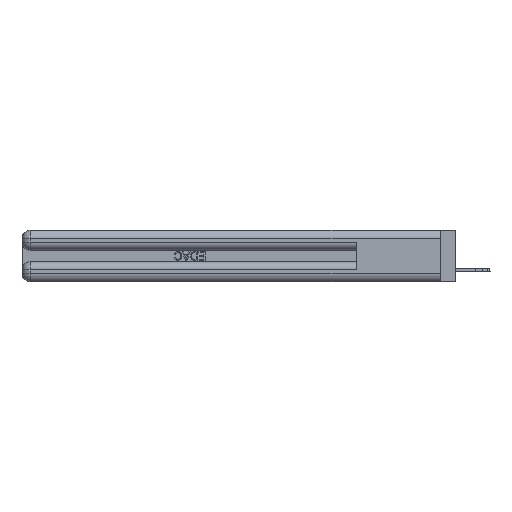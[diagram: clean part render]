
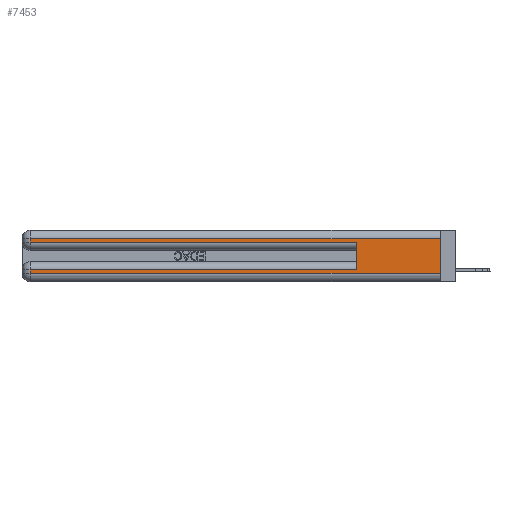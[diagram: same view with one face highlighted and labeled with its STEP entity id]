
A CAD part, left-side view. The second image highlights one B-rep face of the part: STEP entity #7453.
In plain terms, the highlighted planar face has unit normal (-1, 0, 0).
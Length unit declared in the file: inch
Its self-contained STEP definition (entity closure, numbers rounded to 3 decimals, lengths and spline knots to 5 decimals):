
#379 = CARTESIAN_POINT ( 'NONE',  ( 0., 2.94, 0.37 ) ) ;
#559 = VECTOR ( 'NONE', #15615, 39.37008 ) ;
#727 = EDGE_CURVE ( 'NONE', #10303, #22955, #10656, .T. ) ;
#872 = ORIENTED_EDGE ( 'NONE', *, *, #24029, .T. ) ;
#1413 = CARTESIAN_POINT ( 'NONE',  ( 0., 0.6, 0.285 ) ) ;
#3021 = PLANE ( 'NONE',  #16081 ) ;
#3817 = CARTESIAN_POINT ( 'NONE',  ( 0., 0., 0.085 ) ) ;
#3890 = EDGE_CURVE ( 'NONE', #19406, #32691, #26580, .T. ) ;
#3909 = DIRECTION ( 'NONE',  ( 0., 0., -1. ) ) ;
#5257 = LINE ( 'NONE', #3817, #559 ) ;
#7390 = VECTOR ( 'NONE', #3909, 39.37008 ) ;
#7453 = ADVANCED_FACE ( 'NONE', ( #27295 ), #3021, .F. ) ;
#7505 = CARTESIAN_POINT ( 'NONE',  ( 0., 0.6, 0.085 ) ) ;
#8037 = VECTOR ( 'NONE', #27867, 39.37008 ) ;
#9003 = ORIENTED_EDGE ( 'NONE', *, *, #3890, .T. ) ;
#9151 = CARTESIAN_POINT ( 'NONE',  ( 0., 0., 0.37 ) ) ;
#9726 = VECTOR ( 'NONE', #36143, 39.37008 ) ;
#10303 = VERTEX_POINT ( 'NONE', #33658 ) ;
#10656 = LINE ( 'NONE', #9151, #18634 ) ;
#11494 = EDGE_CURVE ( 'NONE', #32691, #19938, #33263, .T. ) ;
#11659 = ORIENTED_EDGE ( 'NONE', *, *, #15062, .F. ) ;
#12539 = DIRECTION ( 'NONE',  ( 0., -1., 0. ) ) ;
#13147 = VECTOR ( 'NONE', #12539, 39.37008 ) ;
#13221 = LINE ( 'NONE', #14712, #25880 ) ;
#13376 = VECTOR ( 'NONE', #16590, 39.37008 ) ;
#14161 = ORIENTED_EDGE ( 'NONE', *, *, #37980, .T. ) ;
#14712 = CARTESIAN_POINT ( 'NONE',  ( 0., 0., 0.06 ) ) ;
#15062 = EDGE_CURVE ( 'NONE', #25900, #19938, #34430, .T. ) ;
#15087 = DIRECTION ( 'NONE',  ( 0., -1., 0. ) ) ;
#15615 = DIRECTION ( 'NONE',  ( 0., 1., 0. ) ) ;
#16004 = LINE ( 'NONE', #30490, #8037 ) ;
#16081 = AXIS2_PLACEMENT_3D ( 'NONE', #18105, #21227, #19192 ) ;
#16102 = CARTESIAN_POINT ( 'NONE',  ( 0., 0., 0.06 ) ) ;
#16590 = DIRECTION ( 'NONE',  ( 0., 0., 1. ) ) ;
#17435 = CARTESIAN_POINT ( 'NONE',  ( 0., 2.94, 0.37 ) ) ;
#18105 = CARTESIAN_POINT ( 'NONE',  ( 0., 0., 0.37 ) ) ;
#18221 = CARTESIAN_POINT ( 'NONE',  ( 0., 2.94, 0.06 ) ) ;
#18634 = VECTOR ( 'NONE', #30602, 39.37008 ) ;
#19192 = DIRECTION ( 'NONE',  ( 0., 0., -1. ) ) ;
#19406 = VERTEX_POINT ( 'NONE', #34688 ) ;
#19938 = VERTEX_POINT ( 'NONE', #1413 ) ;
#21227 = DIRECTION ( 'NONE',  ( 1., 0., 0. ) ) ;
#21993 = CARTESIAN_POINT ( 'NONE',  ( 0., 2.94, 0.285 ) ) ;
#22155 = VERTEX_POINT ( 'NONE', #27006 ) ;
#22955 = VERTEX_POINT ( 'NONE', #16102 ) ;
#24029 = EDGE_CURVE ( 'NONE', #30816, #22955, #13221, .T. ) ;
#24200 = EDGE_CURVE ( 'NONE', #25900, #22155, #5257, .T. ) ;
#25880 = VECTOR ( 'NONE', #15087, 39.37008 ) ;
#25900 = VERTEX_POINT ( 'NONE', #7505 ) ;
#26580 = LINE ( 'NONE', #17435, #9726 ) ;
#26913 = EDGE_CURVE ( 'NONE', #22155, #30816, #35027, .T. ) ;
#27006 = CARTESIAN_POINT ( 'NONE',  ( 0., 2.94, 0.085 ) ) ;
#27295 = FACE_OUTER_BOUND ( 'NONE', #34996, .T. ) ;
#27867 = DIRECTION ( 'NONE',  ( 0., 1., 0. ) ) ;
#29325 = ORIENTED_EDGE ( 'NONE', *, *, #727, .F. ) ;
#30323 = ORIENTED_EDGE ( 'NONE', *, *, #24200, .T. ) ;
#30454 = CARTESIAN_POINT ( 'NONE',  ( 0., 0., 0.285 ) ) ;
#30490 = CARTESIAN_POINT ( 'NONE',  ( 0., 0., 0.31 ) ) ;
#30602 = DIRECTION ( 'NONE',  ( 0., 0., -1. ) ) ;
#30816 = VERTEX_POINT ( 'NONE', #18221 ) ;
#31480 = CARTESIAN_POINT ( 'NONE',  ( 0., 0.6, 0.145 ) ) ;
#32691 = VERTEX_POINT ( 'NONE', #21993 ) ;
#33263 = LINE ( 'NONE', #30454, #13147 ) ;
#33658 = CARTESIAN_POINT ( 'NONE',  ( 0., 0., 0.31 ) ) ;
#34430 = LINE ( 'NONE', #31480, #13376 ) ;
#34688 = CARTESIAN_POINT ( 'NONE',  ( 0., 2.94, 0.31 ) ) ;
#34996 = EDGE_LOOP ( 'NONE', ( #29325, #14161, #9003, #35709, #11659, #30323, #35931, #872 ) ) ;
#35027 = LINE ( 'NONE', #379, #7390 ) ;
#35709 = ORIENTED_EDGE ( 'NONE', *, *, #11494, .T. ) ;
#35931 = ORIENTED_EDGE ( 'NONE', *, *, #26913, .T. ) ;
#36143 = DIRECTION ( 'NONE',  ( 0., 0., -1. ) ) ;
#37980 = EDGE_CURVE ( 'NONE', #10303, #19406, #16004, .T. ) ;
